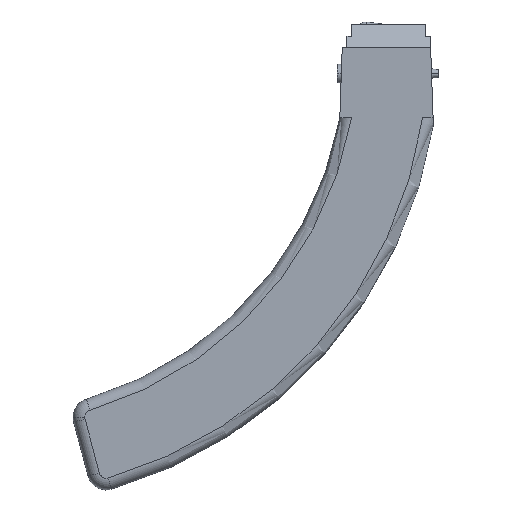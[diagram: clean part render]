
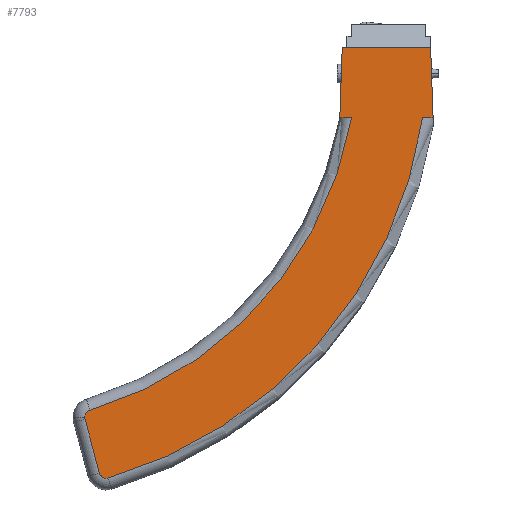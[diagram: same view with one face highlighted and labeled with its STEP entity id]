
A CAD part, top view. The second image highlights one B-rep face of the part: STEP entity #7793.
In plain terms, the highlighted planar face has unit normal (0, 0, 1).
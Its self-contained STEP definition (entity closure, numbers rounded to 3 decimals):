
#42 = PLANE ( 'NONE',  #5197 ) ;
#49 = ORIENTED_EDGE ( 'NONE', *, *, #10682, .T. ) ;
#54 = CARTESIAN_POINT ( 'NONE',  ( 16.349, 2., 16. ) ) ;
#227 = DIRECTION ( 'NONE',  ( 1., 0., 0. ) ) ;
#244 = EDGE_CURVE ( 'NONE', #6622, #2054, #8767, .T. ) ;
#388 = VERTEX_POINT ( 'NONE', #10188 ) ;
#503 = CARTESIAN_POINT ( 'NONE',  ( -131.961, -156.363, 16. ) ) ;
#715 = EDGE_CURVE ( 'NONE', #4278, #11030, #4646, .T. ) ;
#784 = CARTESIAN_POINT ( 'NONE',  ( -128.741, -168.778, 16. ) ) ;
#898 = LINE ( 'NONE', #784, #7623 ) ;
#1122 = VECTOR ( 'NONE', #4044, 1000. ) ;
#1448 = DIRECTION ( 'NONE',  ( 0., 0., 1. ) ) ;
#1507 = ORIENTED_EDGE ( 'NONE', *, *, #10905, .T. ) ;
#1567 = LINE ( 'NONE', #7688, #10608 ) ;
#1658 = DIRECTION ( 'NONE',  ( 0.259, -0.966, 0. ) ) ;
#1867 = VERTEX_POINT ( 'NONE', #54 ) ;
#1981 = AXIS2_PLACEMENT_3D ( 'NONE', #9444, #4209, #10330 ) ;
#2054 = VERTEX_POINT ( 'NONE', #2971 ) ;
#2186 = CIRCLE ( 'NONE', #1981, 190. ) ;
#2354 = ORIENTED_EDGE ( 'NONE', *, *, #9001, .T. ) ;
#2387 = EDGE_CURVE ( 'NONE', #5846, #6349, #4000, .T. ) ;
#2514 = ORIENTED_EDGE ( 'NONE', *, *, #3045, .T. ) ;
#2729 = DIRECTION ( 'NONE',  ( 0., 0., -1. ) ) ;
#2758 = LINE ( 'NONE', #4461, #10304 ) ;
#2836 = CARTESIAN_POINT ( 'NONE',  ( 17.397, -28., 16. ) ) ;
#2863 = EDGE_CURVE ( 'NONE', #4645, #5846, #10087, .T. ) ;
#2971 = CARTESIAN_POINT ( 'NONE',  ( -21.556, 2., 16. ) ) ;
#3012 = CARTESIAN_POINT ( 'NONE',  ( -21.508, 3.359, 16. ) ) ;
#3041 = CARTESIAN_POINT ( 'NONE',  ( -131.859, -157.14, 16. ) ) ;
#3045 = EDGE_CURVE ( 'NONE', #1867, #2054, #10778, .T. ) ;
#3077 = DIRECTION ( 'NONE',  ( -1., 0., 0. ) ) ;
#3101 = CARTESIAN_POINT ( 'NONE',  ( -129.809, -153.485, 16. ) ) ;
#3450 = LINE ( 'NONE', #6667, #1122 ) ;
#3471 = DIRECTION ( 'NONE',  ( 0., 0., 1. ) ) ;
#3892 = AXIS2_PLACEMENT_3D ( 'NONE', #10719, #5464, #227 ) ;
#4000 = CIRCLE ( 'NONE', #9251, 3. ) ;
#4044 = DIRECTION ( 'NONE',  ( -1., 0., 0. ) ) ;
#4157 = EDGE_CURVE ( 'NONE', #6889, #4237, #1567, .T. ) ;
#4209 = DIRECTION ( 'NONE',  ( 0., 0., 1. ) ) ;
#4237 = VERTEX_POINT ( 'NONE', #8686 ) ;
#4254 = CARTESIAN_POINT ( 'NONE',  ( -122.748, -179.552, 16. ) ) ;
#4278 = VERTEX_POINT ( 'NONE', #5238 ) ;
#4358 = ORIENTED_EDGE ( 'NONE', *, *, #2863, .T. ) ;
#4435 = DIRECTION ( 'NONE',  ( 1., 0., 0. ) ) ;
#4461 = CARTESIAN_POINT ( 'NONE',  ( 16.35, 1.963, 16. ) ) ;
#4645 = VERTEX_POINT ( 'NONE', #3101 ) ;
#4646 = CIRCLE ( 'NONE', #8439, 3. ) ;
#5197 = AXIS2_PLACEMENT_3D ( 'NONE', #6172, #9675, #4435 ) ;
#5238 = CARTESIAN_POINT ( 'NONE',  ( -125.646, -180.328, 16. ) ) ;
#5348 = DIRECTION ( 'NONE',  ( -0.035, 0.999, 0. ) ) ;
#5464 = DIRECTION ( 'NONE',  ( 0., 0., 1. ) ) ;
#5759 = ORIENTED_EDGE ( 'NONE', *, *, #715, .T. ) ;
#5846 = VERTEX_POINT ( 'NONE', #503 ) ;
#6172 = CARTESIAN_POINT ( 'NONE',  ( -129.707, -169.037, 16. ) ) ;
#6349 = VERTEX_POINT ( 'NONE', #3041 ) ;
#6622 = VERTEX_POINT ( 'NONE', #10444 ) ;
#6667 = CARTESIAN_POINT ( 'NONE',  ( 17.397, -28., 16. ) ) ;
#6672 = EDGE_CURVE ( 'NONE', #6349, #4278, #898, .T. ) ;
#6731 = VECTOR ( 'NONE', #9112, 1000. ) ;
#6837 = ORIENTED_EDGE ( 'NONE', *, *, #244, .F. ) ;
#6889 = VERTEX_POINT ( 'NONE', #2836 ) ;
#7461 = CARTESIAN_POINT ( 'NONE',  ( 17.397, 2., 16. ) ) ;
#7623 = VECTOR ( 'NONE', #1658, 1000. ) ;
#7641 = CIRCLE ( 'NONE', #9617, 160. ) ;
#7688 = CARTESIAN_POINT ( 'NONE',  ( 17.397, -28., 16. ) ) ;
#7774 = EDGE_LOOP ( 'NONE', ( #49, #11204, #2354, #2514, #6837, #9982, #1507, #4358, #9463, #7858, #5759 ) ) ;
#7793 = ADVANCED_FACE ( 'NONE', ( #10474 ), #42, .T. ) ;
#7858 = ORIENTED_EDGE ( 'NONE', *, *, #6672, .T. ) ;
#7988 = CARTESIAN_POINT ( 'NONE',  ( -175., 0., 16. ) ) ;
#8439 = AXIS2_PLACEMENT_3D ( 'NONE', #4254, #1448, #8617 ) ;
#8574 = DIRECTION ( 'NONE',  ( -1., 0., 0. ) ) ;
#8617 = DIRECTION ( 'NONE',  ( 1., 0., 0. ) ) ;
#8686 = CARTESIAN_POINT ( 'NONE',  ( 12.926, -28., 16. ) ) ;
#8726 = EDGE_CURVE ( 'NONE', #388, #6622, #3450, .T. ) ;
#8729 = CARTESIAN_POINT ( 'NONE',  ( -128.961, -156.363, 16. ) ) ;
#8767 = LINE ( 'NONE', #3012, #6731 ) ;
#8875 = DIRECTION ( 'NONE',  ( 1., 0., 0. ) ) ;
#9001 = EDGE_CURVE ( 'NONE', #6889, #1867, #2758, .T. ) ;
#9112 = DIRECTION ( 'NONE',  ( 0.035, 0.999, 0. ) ) ;
#9251 = AXIS2_PLACEMENT_3D ( 'NONE', #8729, #3471, #9601 ) ;
#9444 = CARTESIAN_POINT ( 'NONE',  ( -175., 0., 16. ) ) ;
#9463 = ORIENTED_EDGE ( 'NONE', *, *, #2387, .T. ) ;
#9601 = DIRECTION ( 'NONE',  ( 1., 0., 0. ) ) ;
#9617 = AXIS2_PLACEMENT_3D ( 'NONE', #7988, #2729, #8875 ) ;
#9675 = DIRECTION ( 'NONE',  ( 0., 0., 1. ) ) ;
#9982 = ORIENTED_EDGE ( 'NONE', *, *, #8726, .F. ) ;
#10087 = CIRCLE ( 'NONE', #3892, 3. ) ;
#10188 = CARTESIAN_POINT ( 'NONE',  ( -17.469, -28., 16. ) ) ;
#10304 = VECTOR ( 'NONE', #5348, 1000. ) ;
#10330 = DIRECTION ( 'NONE',  ( 1., 0., 0. ) ) ;
#10444 = CARTESIAN_POINT ( 'NONE',  ( -22.603, -28., 16. ) ) ;
#10474 = FACE_OUTER_BOUND ( 'NONE', #7774, .T. ) ;
#10503 = VECTOR ( 'NONE', #3077, 1000. ) ;
#10608 = VECTOR ( 'NONE', #8574, 1000. ) ;
#10682 = EDGE_CURVE ( 'NONE', #11030, #4237, #2186, .T. ) ;
#10719 = CARTESIAN_POINT ( 'NONE',  ( -128.961, -156.363, 16. ) ) ;
#10749 = CARTESIAN_POINT ( 'NONE',  ( -121.91, -182.432, 16. ) ) ;
#10778 = LINE ( 'NONE', #7461, #10503 ) ;
#10905 = EDGE_CURVE ( 'NONE', #388, #4645, #7641, .T. ) ;
#11030 = VERTEX_POINT ( 'NONE', #10749 ) ;
#11204 = ORIENTED_EDGE ( 'NONE', *, *, #4157, .F. ) ;
